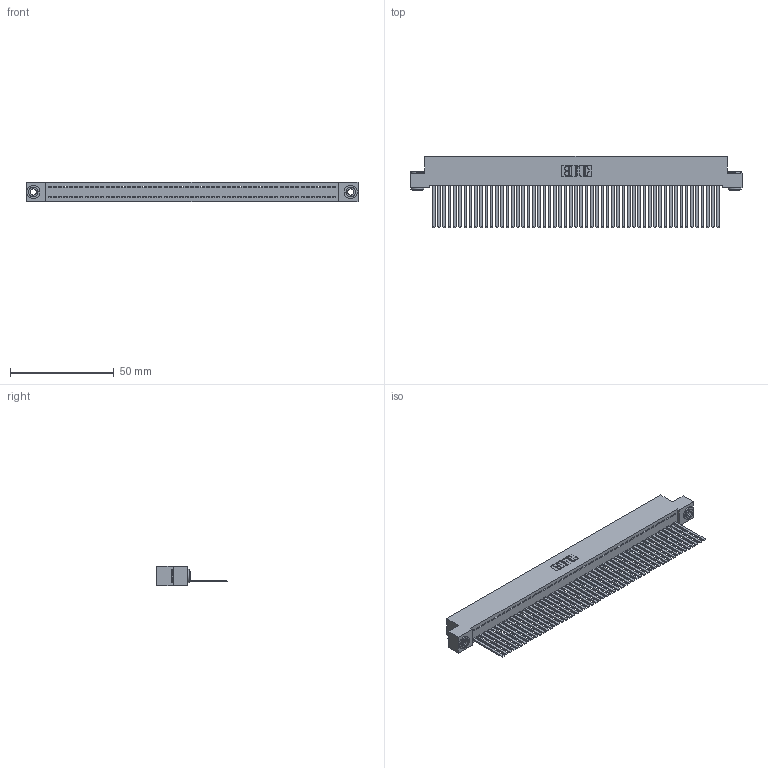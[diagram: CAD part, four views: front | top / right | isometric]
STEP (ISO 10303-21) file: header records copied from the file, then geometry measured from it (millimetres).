
FILE_DESCRIPTION (( 'STEP AP203' ), '1' );
FILE_NAME ('342-055-544-103.STEP', '2019-10-03T04:16:52', ( '' ), ( '' ), 'SwSTEP 2.0', 'SolidWorks 2016', '' );
FILE_SCHEMA (( 'CONFIG_CONTROL_DESIGN' ));
Length unit declared in the file: inch
Products named in the file (4): 342-250-002_345-250-002-102; 342-055-544-103; 342 Part_.156 TH; 345-292-001_345-293-144
Assembly tree (58 placements, depth 2):
  342-055-544-103
    342 Part_.156 TH
    345-292-001_345-293-144  x55
    342-250-002_345-250-002-102  x2
Bounding box: 160.02 x 34.3 x 9.4 mm (x, y, z)
Volume: 14738.2 mm3; surface area: 23924.2 mm2
Topology: 58 solids, 58 shells, 3008 faces, 9065 edges, 5966 vertices
Faces by surface type: plane 2166, cylinder 834, cone 8
Entity records: 32276 total; most frequent: CARTESIAN_POINT 5542, ORIENTED_EDGE 5526, DIRECTION 4679, EDGE_CURVE 2763, VECTOR 2615, LINE 2615, VERTEX_POINT 1838, AXIS2_PLACEMENT_3D 1032
